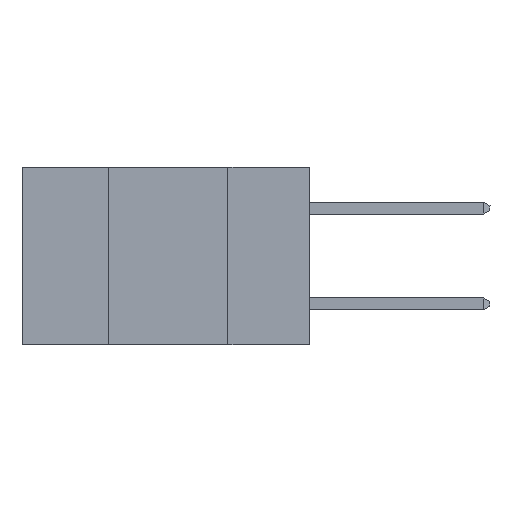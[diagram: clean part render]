
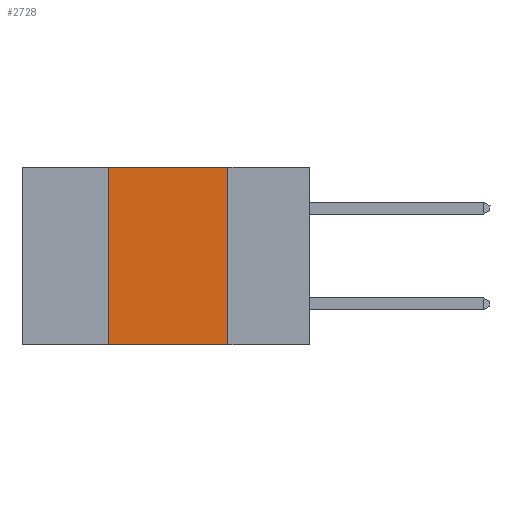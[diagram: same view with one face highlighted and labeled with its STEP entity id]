
A CAD part, left-side view. The second image highlights one B-rep face of the part: STEP entity #2728.
In plain terms, the highlighted planar face has unit normal (-1, 0, 0).
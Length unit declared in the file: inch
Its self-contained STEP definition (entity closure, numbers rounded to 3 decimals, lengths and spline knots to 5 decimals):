
#19 = VECTOR ( 'NONE', #5672, 39.37008 ) ;
#301 = ORIENTED_EDGE ( 'NONE', *, *, #7339, .F. ) ;
#576 = VECTOR ( 'NONE', #1720, 39.37008 ) ;
#1352 = DIRECTION ( 'NONE',  ( 0., 0., -1. ) ) ;
#1720 = DIRECTION ( 'NONE',  ( 0., -1., 0. ) ) ;
#2242 = EDGE_CURVE ( 'NONE', #8976, #7637, #7459, .T. ) ;
#2728 = ADVANCED_FACE ( 'NONE', ( #7933 ), #6228, .F. ) ;
#2917 = CARTESIAN_POINT ( 'NONE',  ( 0., 0.42, -0.37 ) ) ;
#3320 = VECTOR ( 'NONE', #10955, 39.37008 ) ;
#4445 = VERTEX_POINT ( 'NONE', #2917 ) ;
#5233 = CARTESIAN_POINT ( 'NONE',  ( 0., 0.17, -0.37 ) ) ;
#5560 = DIRECTION ( 'NONE',  ( 0., 0., -1. ) ) ;
#5672 = DIRECTION ( 'NONE',  ( 0., 0., 1. ) ) ;
#5745 = DIRECTION ( 'NONE',  ( 1., 0., 0. ) ) ;
#6084 = CARTESIAN_POINT ( 'NONE',  ( 0., 0.6, 0. ) ) ;
#6228 = PLANE ( 'NONE',  #6808 ) ;
#6253 = EDGE_CURVE ( 'NONE', #4445, #8976, #7287, .T. ) ;
#6548 = CARTESIAN_POINT ( 'NONE',  ( 0., 0.42, 0. ) ) ;
#6808 = AXIS2_PLACEMENT_3D ( 'NONE', #6084, #5745, #5560 ) ;
#6961 = ORIENTED_EDGE ( 'NONE', *, *, #2242, .F. ) ;
#7287 = LINE ( 'NONE', #6548, #19 ) ;
#7339 = EDGE_CURVE ( 'NONE', #7637, #10349, #10600, .T. ) ;
#7459 = LINE ( 'NONE', #7789, #576 ) ;
#7637 = VERTEX_POINT ( 'NONE', #7840 ) ;
#7789 = CARTESIAN_POINT ( 'NONE',  ( 0., 0.6, 0. ) ) ;
#7825 = LINE ( 'NONE', #10240, #3320 ) ;
#7840 = CARTESIAN_POINT ( 'NONE',  ( 0., 0.17, 0. ) ) ;
#7933 = FACE_OUTER_BOUND ( 'NONE', #8846, .T. ) ;
#8268 = CARTESIAN_POINT ( 'NONE',  ( 0., 0.17, 0. ) ) ;
#8416 = ORIENTED_EDGE ( 'NONE', *, *, #6253, .F. ) ;
#8593 = VECTOR ( 'NONE', #1352, 39.37008 ) ;
#8657 = CARTESIAN_POINT ( 'NONE',  ( 0., 0.42, 0. ) ) ;
#8846 = EDGE_LOOP ( 'NONE', ( #301, #6961, #8416, #9189 ) ) ;
#8976 = VERTEX_POINT ( 'NONE', #8657 ) ;
#9189 = ORIENTED_EDGE ( 'NONE', *, *, #10520, .T. ) ;
#10240 = CARTESIAN_POINT ( 'NONE',  ( 0., 0.6, -0.37 ) ) ;
#10349 = VERTEX_POINT ( 'NONE', #5233 ) ;
#10520 = EDGE_CURVE ( 'NONE', #4445, #10349, #7825, .T. ) ;
#10600 = LINE ( 'NONE', #8268, #8593 ) ;
#10955 = DIRECTION ( 'NONE',  ( 0., -1., 0. ) ) ;
